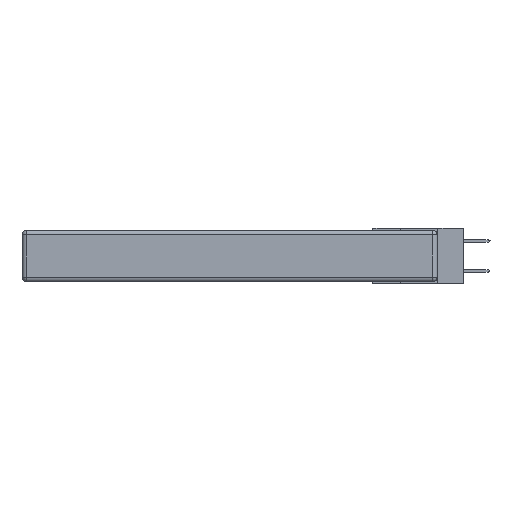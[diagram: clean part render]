
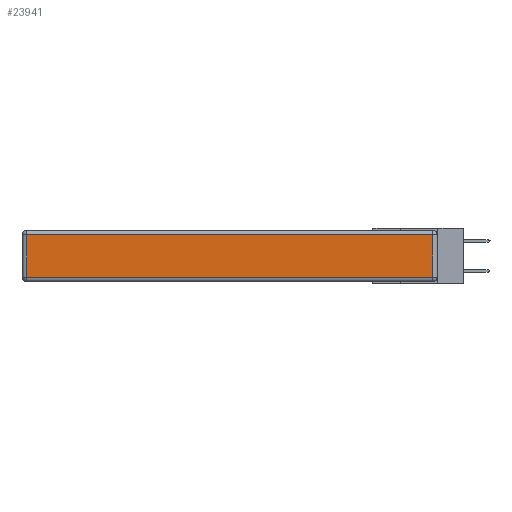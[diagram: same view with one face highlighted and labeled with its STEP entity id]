
A CAD part, left-side view. The second image highlights one B-rep face of the part: STEP entity #23941.
In plain terms, the highlighted planar face has unit normal (-1, 0, 0).
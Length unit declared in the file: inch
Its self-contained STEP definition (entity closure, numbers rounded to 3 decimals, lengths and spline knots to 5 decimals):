
#566 = EDGE_LOOP ( 'NONE', ( #19067, #4248, #3705, #26062 ) ) ;
#2586 = CARTESIAN_POINT ( 'NONE',  ( 0., 0.03, -0.343 ) ) ;
#3705 = ORIENTED_EDGE ( 'NONE', *, *, #22012, .T. ) ;
#4051 = LINE ( 'NONE', #16780, #21498 ) ;
#4248 = ORIENTED_EDGE ( 'NONE', *, *, #10016, .T. ) ;
#4513 = CARTESIAN_POINT ( 'NONE',  ( 0., 0.03, -0.03 ) ) ;
#5552 = LINE ( 'NONE', #23356, #16928 ) ;
#6292 = DIRECTION ( 'NONE',  ( 0., 0., 1. ) ) ;
#6573 = VERTEX_POINT ( 'NONE', #4513 ) ;
#8272 = CARTESIAN_POINT ( 'NONE',  ( 0., 0., -0.343 ) ) ;
#8384 = DIRECTION ( 'NONE',  ( 0., 0., -1. ) ) ;
#9032 = LINE ( 'NONE', #2586, #13086 ) ;
#9095 = CARTESIAN_POINT ( 'NONE',  ( 0., 2.75, -0.03 ) ) ;
#10016 = EDGE_CURVE ( 'NONE', #10347, #6573, #9032, .T. ) ;
#10347 = VERTEX_POINT ( 'NONE', #22177 ) ;
#13086 = VECTOR ( 'NONE', #26752, 39.37008 ) ;
#14058 = EDGE_CURVE ( 'NONE', #28098, #10347, #5552, .T. ) ;
#16780 = CARTESIAN_POINT ( 'NONE',  ( 0., 2.72, -0.343 ) ) ;
#16928 = VECTOR ( 'NONE', #20638, 39.37008 ) ;
#18480 = PLANE ( 'NONE',  #21635 ) ;
#19067 = ORIENTED_EDGE ( 'NONE', *, *, #14058, .T. ) ;
#20638 = DIRECTION ( 'NONE',  ( 0., -1., 0. ) ) ;
#21498 = VECTOR ( 'NONE', #8384, 39.37008 ) ;
#21635 = AXIS2_PLACEMENT_3D ( 'NONE', #8272, #26872, #6292 ) ;
#22012 = EDGE_CURVE ( 'NONE', #6573, #26483, #22699, .T. ) ;
#22177 = CARTESIAN_POINT ( 'NONE',  ( 0., 0.03, -0.313 ) ) ;
#22699 = LINE ( 'NONE', #9095, #32073 ) ;
#22778 = CARTESIAN_POINT ( 'NONE',  ( 0., 2.72, -0.03 ) ) ;
#23356 = CARTESIAN_POINT ( 'NONE',  ( 0., 0., -0.313 ) ) ;
#23941 = ADVANCED_FACE ( 'NONE', ( #31921 ), #18480, .T. ) ;
#24288 = DIRECTION ( 'NONE',  ( 0., 1., 0. ) ) ;
#26062 = ORIENTED_EDGE ( 'NONE', *, *, #28236, .T. ) ;
#26483 = VERTEX_POINT ( 'NONE', #22778 ) ;
#26752 = DIRECTION ( 'NONE',  ( 0., 0., 1. ) ) ;
#26872 = DIRECTION ( 'NONE',  ( -1., 0., 0. ) ) ;
#28098 = VERTEX_POINT ( 'NONE', #30775 ) ;
#28236 = EDGE_CURVE ( 'NONE', #26483, #28098, #4051, .T. ) ;
#30775 = CARTESIAN_POINT ( 'NONE',  ( 0., 2.72, -0.313 ) ) ;
#31921 = FACE_OUTER_BOUND ( 'NONE', #566, .T. ) ;
#32073 = VECTOR ( 'NONE', #24288, 39.37008 ) ;
